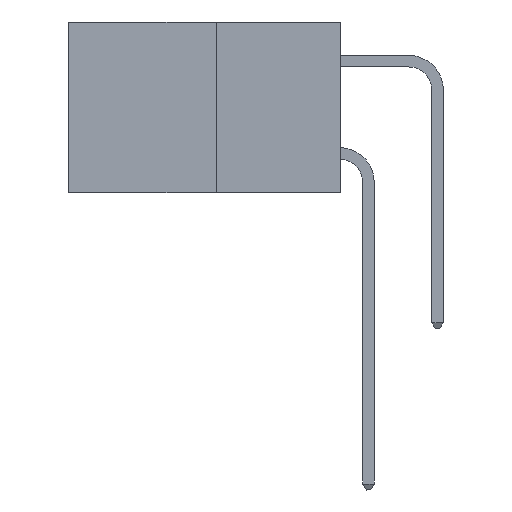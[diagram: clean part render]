
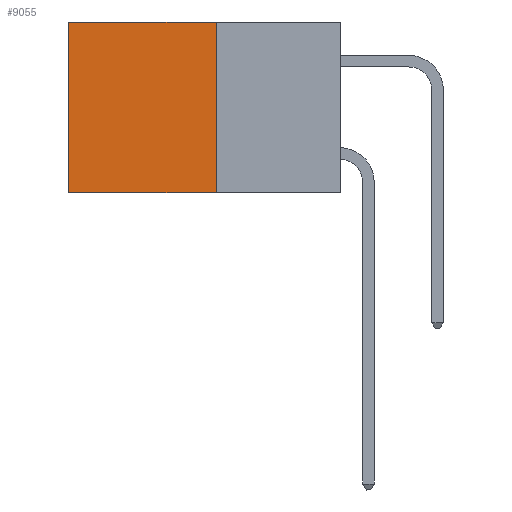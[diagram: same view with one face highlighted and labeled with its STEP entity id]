
A CAD part, left-side view. The second image highlights one B-rep face of the part: STEP entity #9055.
In plain terms, the highlighted planar face has unit normal (-1, 0, 0).
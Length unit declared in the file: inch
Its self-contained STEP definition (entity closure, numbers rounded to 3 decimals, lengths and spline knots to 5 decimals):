
#461 = VERTEX_POINT ( 'NONE', #13329 ) ;
#531 = CARTESIAN_POINT ( 'NONE',  ( 0.277, 0.27, 0. ) ) ;
#643 = EDGE_CURVE ( 'NONE', #8881, #14202, #14518, .T. ) ;
#1569 = DIRECTION ( 'NONE',  ( 0., 1., 0. ) ) ;
#1666 = VECTOR ( 'NONE', #6472, 39.37008 ) ;
#1941 = DIRECTION ( 'NONE',  ( 0., 0., -1. ) ) ;
#2286 = EDGE_CURVE ( 'NONE', #9499, #461, #11169, .T. ) ;
#2460 = CARTESIAN_POINT ( 'NONE',  ( 0.277, 0.27, -0.37 ) ) ;
#2565 = CARTESIAN_POINT ( 'NONE',  ( 0.277, 0.27, 0. ) ) ;
#4115 = ORIENTED_EDGE ( 'NONE', *, *, #10322, .F. ) ;
#4811 = PLANE ( 'NONE',  #15366 ) ;
#5193 = LINE ( 'NONE', #2460, #1666 ) ;
#5311 = CARTESIAN_POINT ( 'NONE',  ( 0.277, 0.27, -0.37 ) ) ;
#5348 = CARTESIAN_POINT ( 'NONE',  ( 0.277, 0.27, -0.37 ) ) ;
#6413 = ORIENTED_EDGE ( 'NONE', *, *, #8508, .T. ) ;
#6472 = DIRECTION ( 'NONE',  ( 0., 0., -1. ) ) ;
#6753 = CARTESIAN_POINT ( 'NONE',  ( 0.277, 0.59, 0. ) ) ;
#7081 = DIRECTION ( 'NONE',  ( 1., 0., 0. ) ) ;
#7661 = VECTOR ( 'NONE', #12051, 39.37008 ) ;
#7844 = EDGE_LOOP ( 'NONE', ( #6413, #13222, #4115, #7986 ) ) ;
#7986 = ORIENTED_EDGE ( 'NONE', *, *, #643, .T. ) ;
#7997 = CARTESIAN_POINT ( 'NONE',  ( 0.277, 0.27, -0.37 ) ) ;
#8508 = EDGE_CURVE ( 'NONE', #14202, #461, #12294, .T. ) ;
#8881 = VERTEX_POINT ( 'NONE', #2565 ) ;
#9055 = ADVANCED_FACE ( 'NONE', ( #13930 ), #4811, .F. ) ;
#9492 = DIRECTION ( 'NONE',  ( 0., 0., -1. ) ) ;
#9499 = VERTEX_POINT ( 'NONE', #5348 ) ;
#10322 = EDGE_CURVE ( 'NONE', #8881, #9499, #5193, .T. ) ;
#11169 = LINE ( 'NONE', #7997, #14270 ) ;
#12051 = DIRECTION ( 'NONE',  ( 0., 1., 0. ) ) ;
#12294 = LINE ( 'NONE', #15956, #16167 ) ;
#13222 = ORIENTED_EDGE ( 'NONE', *, *, #2286, .F. ) ;
#13329 = CARTESIAN_POINT ( 'NONE',  ( 0.277, 0.59, -0.37 ) ) ;
#13930 = FACE_OUTER_BOUND ( 'NONE', #7844, .T. ) ;
#14202 = VERTEX_POINT ( 'NONE', #6753 ) ;
#14270 = VECTOR ( 'NONE', #1569, 39.37008 ) ;
#14518 = LINE ( 'NONE', #531, #7661 ) ;
#15366 = AXIS2_PLACEMENT_3D ( 'NONE', #5311, #7081, #9492 ) ;
#15956 = CARTESIAN_POINT ( 'NONE',  ( 0.277, 0.59, -0.37 ) ) ;
#16167 = VECTOR ( 'NONE', #1941, 39.37008 ) ;
